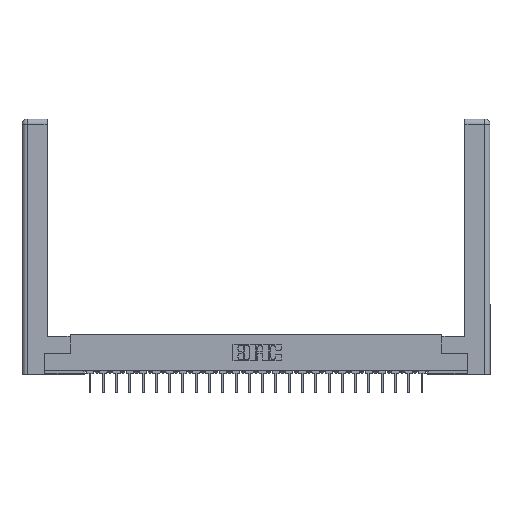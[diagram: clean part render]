
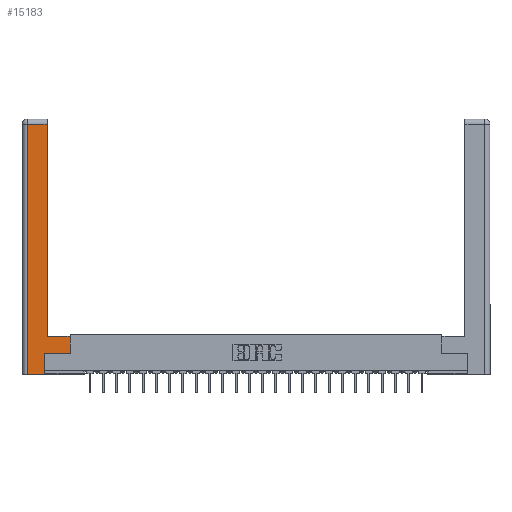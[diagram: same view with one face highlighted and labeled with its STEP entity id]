
A CAD part, top view. The second image highlights one B-rep face of the part: STEP entity #15183.
In plain terms, the highlighted planar face has unit normal (0, 0, 1).
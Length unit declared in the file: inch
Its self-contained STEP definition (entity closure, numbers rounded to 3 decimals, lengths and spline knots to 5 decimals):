
#40 = LINE ( 'NONE', #13887, #8094 ) ;
#113 = CARTESIAN_POINT ( 'NONE',  ( 0.265, 0., 0. ) ) ;
#115 = ORIENTED_EDGE ( 'NONE', *, *, #2841, .T. ) ;
#233 = EDGE_CURVE ( 'NONE', #4717, #18770, #25016, .T. ) ;
#424 = ORIENTED_EDGE ( 'NONE', *, *, #453, .T. ) ;
#453 = EDGE_CURVE ( 'NONE', #12423, #19872, #11611, .T. ) ;
#893 = LINE ( 'NONE', #11552, #12576 ) ;
#1879 = VERTEX_POINT ( 'NONE', #19265 ) ;
#2285 = DIRECTION ( 'NONE',  ( 1., 0., 0. ) ) ;
#2841 = EDGE_CURVE ( 'NONE', #1879, #6142, #24500, .T. ) ;
#3307 = CARTESIAN_POINT ( 'NONE',  ( 0.295, 3., 0. ) ) ;
#3376 = VECTOR ( 'NONE', #20199, 39.37008 ) ;
#3592 = EDGE_LOOP ( 'NONE', ( #13373, #424, #9430, #115, #15355, #19228, #26194, #24631 ) ) ;
#4400 = CARTESIAN_POINT ( 'NONE',  ( 0.565, 0.45, 0. ) ) ;
#4717 = VERTEX_POINT ( 'NONE', #5077 ) ;
#5077 = CARTESIAN_POINT ( 'NONE',  ( 0.565, 0.245, 0. ) ) ;
#5676 = CARTESIAN_POINT ( 'NONE',  ( 0.0615, 2.94, 0. ) ) ;
#6142 = VERTEX_POINT ( 'NONE', #14270 ) ;
#6744 = LINE ( 'NONE', #19927, #23770 ) ;
#7185 = EDGE_CURVE ( 'NONE', #19872, #1879, #893, .T. ) ;
#7372 = DIRECTION ( 'NONE',  ( 0., -1., 0. ) ) ;
#7800 = DIRECTION ( 'NONE',  ( 0., 1., 0. ) ) ;
#8005 = DIRECTION ( 'NONE',  ( -1., 0., 0. ) ) ;
#8094 = VECTOR ( 'NONE', #20245, 39.37008 ) ;
#8507 = AXIS2_PLACEMENT_3D ( 'NONE', #15909, #22265, #22358 ) ;
#9361 = VERTEX_POINT ( 'NONE', #14432 ) ;
#9430 = ORIENTED_EDGE ( 'NONE', *, *, #7185, .T. ) ;
#10406 = LINE ( 'NONE', #24343, #3376 ) ;
#11293 = EDGE_CURVE ( 'NONE', #15543, #12423, #26401, .T. ) ;
#11552 = CARTESIAN_POINT ( 'NONE',  ( 0.0615, 0., 0. ) ) ;
#11611 = LINE ( 'NONE', #25005, #15918 ) ;
#12423 = VERTEX_POINT ( 'NONE', #22862 ) ;
#12576 = VECTOR ( 'NONE', #7372, 39.37008 ) ;
#12848 = DIRECTION ( 'NONE',  ( 0., 1., 0. ) ) ;
#13373 = ORIENTED_EDGE ( 'NONE', *, *, #11293, .T. ) ;
#13461 = CARTESIAN_POINT ( 'NONE',  ( 0.295, 0.45, 0. ) ) ;
#13887 = CARTESIAN_POINT ( 'NONE',  ( 0.265, 0.245, 0. ) ) ;
#14270 = CARTESIAN_POINT ( 'NONE',  ( 0.265, 0., 0. ) ) ;
#14432 = CARTESIAN_POINT ( 'NONE',  ( 0.265, 0.245, 0. ) ) ;
#15183 = ADVANCED_FACE ( 'NONE', ( #24625 ), #17987, .F. ) ;
#15355 = ORIENTED_EDGE ( 'NONE', *, *, #21565, .T. ) ;
#15543 = VERTEX_POINT ( 'NONE', #13461 ) ;
#15909 = CARTESIAN_POINT ( 'NONE',  ( 0., 0., 0. ) ) ;
#15918 = VECTOR ( 'NONE', #8005, 39.37008 ) ;
#17280 = VECTOR ( 'NONE', #12848, 39.37008 ) ;
#17987 = PLANE ( 'NONE',  #8507 ) ;
#18669 = VECTOR ( 'NONE', #7800, 39.37008 ) ;
#18770 = VERTEX_POINT ( 'NONE', #4400 ) ;
#19228 = ORIENTED_EDGE ( 'NONE', *, *, #26818, .T. ) ;
#19265 = CARTESIAN_POINT ( 'NONE',  ( 0.0615, 0., 0. ) ) ;
#19872 = VERTEX_POINT ( 'NONE', #5676 ) ;
#19927 = CARTESIAN_POINT ( 'NONE',  ( 0.295, 0.45, 0. ) ) ;
#20103 = DIRECTION ( 'NONE',  ( -1., 0., 0. ) ) ;
#20199 = DIRECTION ( 'NONE',  ( 1., 0., 0. ) ) ;
#20245 = DIRECTION ( 'NONE',  ( 0., 1., 0. ) ) ;
#21565 = EDGE_CURVE ( 'NONE', #6142, #9361, #40, .T. ) ;
#22265 = DIRECTION ( 'NONE',  ( 0., 0., -1. ) ) ;
#22358 = DIRECTION ( 'NONE',  ( -1., 0., 0. ) ) ;
#22862 = CARTESIAN_POINT ( 'NONE',  ( 0.295, 2.94, 0. ) ) ;
#23770 = VECTOR ( 'NONE', #20103, 39.37008 ) ;
#23831 = VECTOR ( 'NONE', #2285, 39.37008 ) ;
#24343 = CARTESIAN_POINT ( 'NONE',  ( 0.565, 0.245, 0. ) ) ;
#24500 = LINE ( 'NONE', #113, #23831 ) ;
#24625 = FACE_OUTER_BOUND ( 'NONE', #3592, .T. ) ;
#24631 = ORIENTED_EDGE ( 'NONE', *, *, #26859, .T. ) ;
#25005 = CARTESIAN_POINT ( 'NONE',  ( 0.0615, 2.94, 0. ) ) ;
#25016 = LINE ( 'NONE', #25678, #17280 ) ;
#25678 = CARTESIAN_POINT ( 'NONE',  ( 0.565, 0.45, 0. ) ) ;
#26194 = ORIENTED_EDGE ( 'NONE', *, *, #233, .T. ) ;
#26401 = LINE ( 'NONE', #3307, #18669 ) ;
#26818 = EDGE_CURVE ( 'NONE', #9361, #4717, #10406, .T. ) ;
#26859 = EDGE_CURVE ( 'NONE', #18770, #15543, #6744, .T. ) ;
